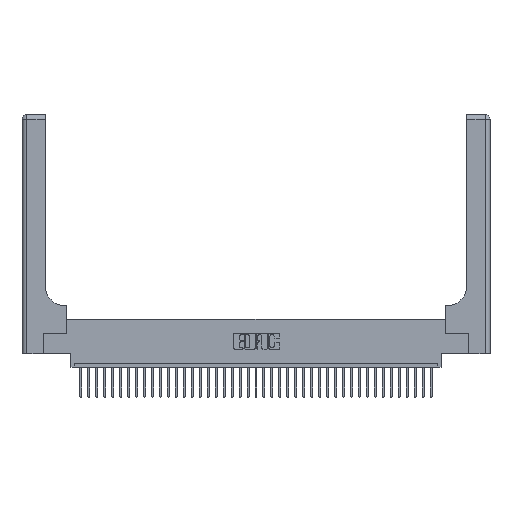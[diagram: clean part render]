
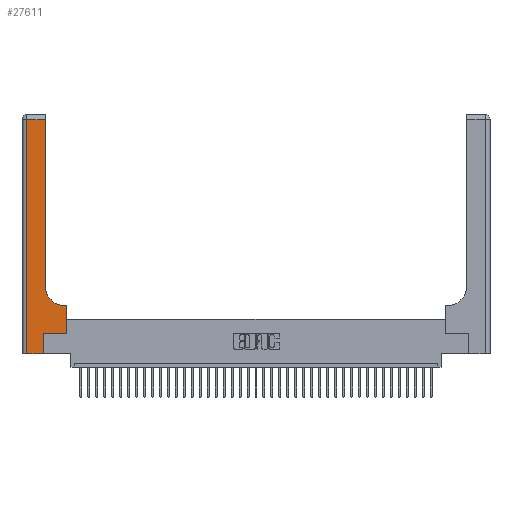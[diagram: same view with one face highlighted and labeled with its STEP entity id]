
A CAD part, top view. The second image highlights one B-rep face of the part: STEP entity #27611.
In plain terms, the highlighted planar face has unit normal (0, 0, 1).
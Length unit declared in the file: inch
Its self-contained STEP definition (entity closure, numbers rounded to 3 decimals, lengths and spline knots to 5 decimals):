
#30 = CARTESIAN_POINT ( 'NONE',  ( 0.5585, 0.6, 0.37 ) ) ;
#343 = CARTESIAN_POINT ( 'NONE',  ( 0.06, 0., 0.37 ) ) ;
#483 = LINE ( 'NONE', #31751, #28117 ) ;
#1562 = DIRECTION ( 'NONE',  ( 0., 1., 0. ) ) ;
#1802 = CARTESIAN_POINT ( 'NONE',  ( 0.269, 0., 0.37 ) ) ;
#1856 = ORIENTED_EDGE ( 'NONE', *, *, #15823, .T. ) ;
#1940 = CARTESIAN_POINT ( 'NONE',  ( 0.5585, 0.25, 0.37 ) ) ;
#2582 = CARTESIAN_POINT ( 'NONE',  ( 0.2915, 2.94, 0.37 ) ) ;
#2589 = EDGE_CURVE ( 'NONE', #16618, #23311, #9248, .T. ) ;
#2621 = CARTESIAN_POINT ( 'NONE',  ( 0., 2.94, 0.37 ) ) ;
#3069 = DIRECTION ( 'NONE',  ( 1., 0., 0. ) ) ;
#4249 = EDGE_CURVE ( 'NONE', #23311, #9884, #28243, .T. ) ;
#4309 = CARTESIAN_POINT ( 'NONE',  ( 0.2915, 3., 0.37 ) ) ;
#4739 = CARTESIAN_POINT ( 'NONE',  ( 0.269, 0., 0.37 ) ) ;
#4797 = VERTEX_POINT ( 'NONE', #30 ) ;
#4890 = LINE ( 'NONE', #38265, #14646 ) ;
#5528 = VECTOR ( 'NONE', #7187, 39.37008 ) ;
#5672 = EDGE_LOOP ( 'NONE', ( #5846, #28248, #1856, #10122, #16699, #8161, #20696, #27848, #25200 ) ) ;
#5846 = ORIENTED_EDGE ( 'NONE', *, *, #2589, .T. ) ;
#6678 = VECTOR ( 'NONE', #26238, 39.37008 ) ;
#7172 = EDGE_CURVE ( 'NONE', #14536, #12914, #24227, .T. ) ;
#7187 = DIRECTION ( 'NONE',  ( 0., 1., 0. ) ) ;
#7581 = VERTEX_POINT ( 'NONE', #343 ) ;
#7647 = CARTESIAN_POINT ( 'NONE',  ( 0.06, 3., 0.37 ) ) ;
#7720 = CARTESIAN_POINT ( 'NONE',  ( 0.5415, 0.6, 0.37 ) ) ;
#8161 = ORIENTED_EDGE ( 'NONE', *, *, #7172, .T. ) ;
#9248 = LINE ( 'NONE', #4309, #5528 ) ;
#9884 = VERTEX_POINT ( 'NONE', #12369 ) ;
#10122 = ORIENTED_EDGE ( 'NONE', *, *, #20194, .T. ) ;
#10210 = EDGE_CURVE ( 'NONE', #12914, #4797, #30536, .T. ) ;
#10940 = AXIS2_PLACEMENT_3D ( 'NONE', #11053, #32423, #22971 ) ;
#11053 = CARTESIAN_POINT ( 'NONE',  ( 0.5415, 0.85, 0.37 ) ) ;
#11140 = DIRECTION ( 'NONE',  ( 1., 0., 0. ) ) ;
#11313 = EDGE_CURVE ( 'NONE', #4797, #29518, #483, .T. ) ;
#12369 = CARTESIAN_POINT ( 'NONE',  ( 0.06, 2.94, 0.37 ) ) ;
#12591 = CARTESIAN_POINT ( 'NONE',  ( 0.5585, 0.25, 0.37 ) ) ;
#12914 = VERTEX_POINT ( 'NONE', #12591 ) ;
#13114 = VECTOR ( 'NONE', #34332, 39.37008 ) ;
#13537 = VERTEX_POINT ( 'NONE', #1802 ) ;
#14315 = VECTOR ( 'NONE', #1562, 39.37008 ) ;
#14536 = VERTEX_POINT ( 'NONE', #20036 ) ;
#14646 = VECTOR ( 'NONE', #11140, 39.37008 ) ;
#14773 = CARTESIAN_POINT ( 'NONE',  ( 0.269, 0.25, 0.37 ) ) ;
#15823 = EDGE_CURVE ( 'NONE', #9884, #7581, #37036, .T. ) ;
#16618 = VERTEX_POINT ( 'NONE', #34984 ) ;
#16699 = ORIENTED_EDGE ( 'NONE', *, *, #32469, .T. ) ;
#19317 = VECTOR ( 'NONE', #23516, 39.37008 ) ;
#19950 = DIRECTION ( 'NONE',  ( -1., 0., 0. ) ) ;
#20036 = CARTESIAN_POINT ( 'NONE',  ( 0.269, 0.25, 0.37 ) ) ;
#20194 = EDGE_CURVE ( 'NONE', #7581, #13537, #4890, .T. ) ;
#20696 = ORIENTED_EDGE ( 'NONE', *, *, #10210, .T. ) ;
#22464 = CARTESIAN_POINT ( 'NONE',  ( 0., 3., 0.37 ) ) ;
#22674 = DIRECTION ( 'NONE',  ( -1., 0., 0. ) ) ;
#22914 = EDGE_CURVE ( 'NONE', #29518, #16618, #22936, .T. ) ;
#22936 = CIRCLE ( 'NONE', #10940, 0.25 ) ;
#22971 = DIRECTION ( 'NONE',  ( 1., 0., 0. ) ) ;
#22995 = DIRECTION ( 'NONE',  ( 0., 0., -1. ) ) ;
#23311 = VERTEX_POINT ( 'NONE', #2582 ) ;
#23516 = DIRECTION ( 'NONE',  ( -1., 0., 0. ) ) ;
#24227 = LINE ( 'NONE', #14773, #29389 ) ;
#25200 = ORIENTED_EDGE ( 'NONE', *, *, #22914, .T. ) ;
#26238 = DIRECTION ( 'NONE',  ( 0., 1., 0. ) ) ;
#26383 = FACE_OUTER_BOUND ( 'NONE', #5672, .T. ) ;
#27611 = ADVANCED_FACE ( 'NONE', ( #26383 ), #28351, .F. ) ;
#27848 = ORIENTED_EDGE ( 'NONE', *, *, #11313, .T. ) ;
#28117 = VECTOR ( 'NONE', #22674, 39.37008 ) ;
#28243 = LINE ( 'NONE', #2621, #19317 ) ;
#28248 = ORIENTED_EDGE ( 'NONE', *, *, #4249, .T. ) ;
#28351 = PLANE ( 'NONE',  #36219 ) ;
#29389 = VECTOR ( 'NONE', #3069, 39.37008 ) ;
#29518 = VERTEX_POINT ( 'NONE', #7720 ) ;
#30290 = LINE ( 'NONE', #4739, #14315 ) ;
#30536 = LINE ( 'NONE', #1940, #6678 ) ;
#31751 = CARTESIAN_POINT ( 'NONE',  ( 0.2915, 0.6, 0.37 ) ) ;
#32423 = DIRECTION ( 'NONE',  ( 0., 0., -1. ) ) ;
#32469 = EDGE_CURVE ( 'NONE', #13537, #14536, #30290, .T. ) ;
#34332 = DIRECTION ( 'NONE',  ( 0., -1., 0. ) ) ;
#34984 = CARTESIAN_POINT ( 'NONE',  ( 0.2915, 0.85, 0.37 ) ) ;
#36219 = AXIS2_PLACEMENT_3D ( 'NONE', #22464, #22995, #19950 ) ;
#37036 = LINE ( 'NONE', #7647, #13114 ) ;
#38265 = CARTESIAN_POINT ( 'NONE',  ( 0., 0., 0.37 ) ) ;
